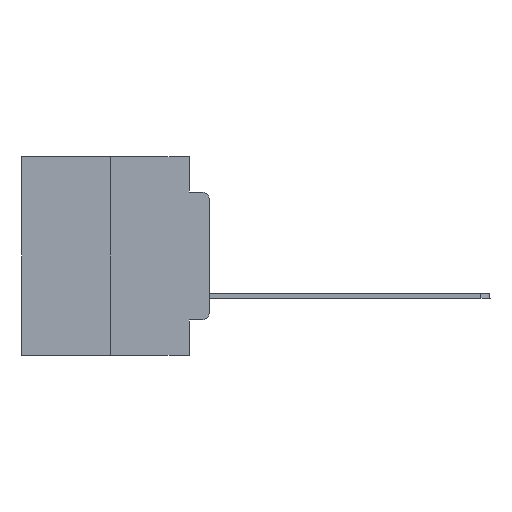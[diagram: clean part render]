
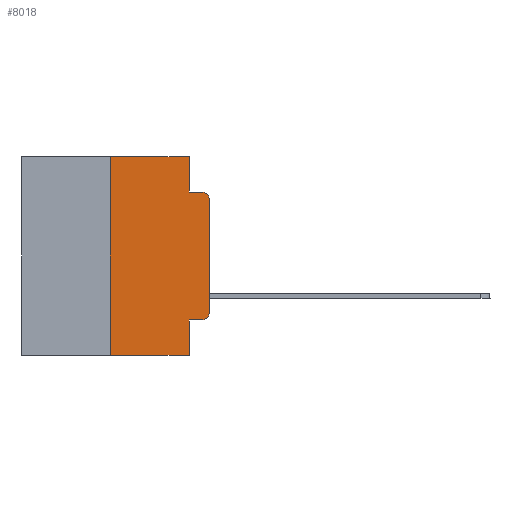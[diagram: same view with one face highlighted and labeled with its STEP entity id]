
A CAD part, left-side view. The second image highlights one B-rep face of the part: STEP entity #8018.
In plain terms, the highlighted planar face has unit normal (-1, 0, 0).
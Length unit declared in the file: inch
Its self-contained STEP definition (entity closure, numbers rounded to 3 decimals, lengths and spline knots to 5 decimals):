
#110 = LINE ( 'NONE', #20699, #1363 ) ;
#920 = EDGE_LOOP ( 'NONE', ( #15787, #13832, #15679, #2842, #12785, #22936, #7145, #8000, #10165, #6004 ) ) ;
#1363 = VECTOR ( 'NONE', #5679, 39.37008 ) ;
#1637 = DIRECTION ( 'NONE',  ( 0., 0., 1. ) ) ;
#1907 = EDGE_CURVE ( 'NONE', #15373, #3671, #4160, .T. ) ;
#2144 = CARTESIAN_POINT ( 'NONE',  ( 0., 0.02, -0.0885 ) ) ;
#2605 = CARTESIAN_POINT ( 'NONE',  ( 0., 0.02, -0.4115 ) ) ;
#2620 = CARTESIAN_POINT ( 'NONE',  ( 0., 0.051, -0.0885 ) ) ;
#2698 = VECTOR ( 'NONE', #14710, 39.37008 ) ;
#2842 = ORIENTED_EDGE ( 'NONE', *, *, #9728, .F. ) ;
#3425 = VERTEX_POINT ( 'NONE', #2605 ) ;
#3671 = VERTEX_POINT ( 'NONE', #13565 ) ;
#4160 = LINE ( 'NONE', #23422, #6907 ) ;
#4455 = VERTEX_POINT ( 'NONE', #24494 ) ;
#4580 = DIRECTION ( 'NONE',  ( 0., -1., 0. ) ) ;
#4675 = VECTOR ( 'NONE', #8907, 39.37008 ) ;
#4723 = DIRECTION ( 'NONE',  ( 0., -1., 0. ) ) ;
#4788 = VERTEX_POINT ( 'NONE', #14912 ) ;
#4839 = AXIS2_PLACEMENT_3D ( 'NONE', #7687, #7604, #5949 ) ;
#5307 = LINE ( 'NONE', #22764, #11201 ) ;
#5679 = DIRECTION ( 'NONE',  ( 0., 0., -1. ) ) ;
#5792 = CARTESIAN_POINT ( 'NONE',  ( 0., 0.25, -0.5 ) ) ;
#5949 = DIRECTION ( 'NONE',  ( 0., 0., -1. ) ) ;
#6004 = ORIENTED_EDGE ( 'NONE', *, *, #6723, .T. ) ;
#6352 = CARTESIAN_POINT ( 'NONE',  ( 0., 0.051, -0.4115 ) ) ;
#6611 = CARTESIAN_POINT ( 'NONE',  ( 0., 0.473, 0. ) ) ;
#6723 = EDGE_CURVE ( 'NONE', #3425, #19789, #13620, .T. ) ;
#6907 = VECTOR ( 'NONE', #13314, 39.37008 ) ;
#7145 = ORIENTED_EDGE ( 'NONE', *, *, #1907, .T. ) ;
#7290 = LINE ( 'NONE', #14428, #11926 ) ;
#7604 = DIRECTION ( 'NONE',  ( -1., 0., 0. ) ) ;
#7687 = CARTESIAN_POINT ( 'NONE',  ( 0., 0.02, -0.3915 ) ) ;
#8000 = ORIENTED_EDGE ( 'NONE', *, *, #24220, .F. ) ;
#8018 = ADVANCED_FACE ( 'NONE', ( #23528 ), #16498, .F. ) ;
#8704 = DIRECTION ( 'NONE',  ( 0., 0., -1. ) ) ;
#8907 = DIRECTION ( 'NONE',  ( 0., 0., 1. ) ) ;
#9728 = EDGE_CURVE ( 'NONE', #21438, #4788, #5307, .T. ) ;
#10165 = ORIENTED_EDGE ( 'NONE', *, *, #18869, .T. ) ;
#10586 = CARTESIAN_POINT ( 'NONE',  ( 0., 0.051, 0. ) ) ;
#10835 = DIRECTION ( 'NONE',  ( 0., 0., -1. ) ) ;
#10953 = CARTESIAN_POINT ( 'NONE',  ( 0., 0.25, 0. ) ) ;
#10961 = CARTESIAN_POINT ( 'NONE',  ( 0., 0., -0.3915 ) ) ;
#11027 = CARTESIAN_POINT ( 'NONE',  ( 0., 0., -0.1085 ) ) ;
#11164 = CARTESIAN_POINT ( 'NONE',  ( 0., 0.02, -0.1085 ) ) ;
#11201 = VECTOR ( 'NONE', #10835, 39.37008 ) ;
#11926 = VECTOR ( 'NONE', #4723, 39.37008 ) ;
#12785 = ORIENTED_EDGE ( 'NONE', *, *, #19736, .F. ) ;
#13314 = DIRECTION ( 'NONE',  ( 0., -1., 0. ) ) ;
#13565 = CARTESIAN_POINT ( 'NONE',  ( 0., 0.051, -0.5 ) ) ;
#13620 = CIRCLE ( 'NONE', #4839, 0.02 ) ;
#13832 = ORIENTED_EDGE ( 'NONE', *, *, #16430, .T. ) ;
#14428 = CARTESIAN_POINT ( 'NONE',  ( 0., 0.473, 0. ) ) ;
#14657 = CARTESIAN_POINT ( 'NONE',  ( 0., 0.25, 0. ) ) ;
#14710 = DIRECTION ( 'NONE',  ( 0., -1., 0. ) ) ;
#14853 = EDGE_CURVE ( 'NONE', #4788, #22424, #18053, .T. ) ;
#14912 = CARTESIAN_POINT ( 'NONE',  ( 0., 0.051, -0.0885 ) ) ;
#15373 = VERTEX_POINT ( 'NONE', #5792 ) ;
#15411 = DIRECTION ( 'NONE',  ( 0., 0., -1. ) ) ;
#15679 = ORIENTED_EDGE ( 'NONE', *, *, #14853, .F. ) ;
#15787 = ORIENTED_EDGE ( 'NONE', *, *, #25307, .T. ) ;
#16184 = VECTOR ( 'NONE', #1637, 39.37008 ) ;
#16346 = EDGE_CURVE ( 'NONE', #15373, #22776, #23337, .T. ) ;
#16430 = EDGE_CURVE ( 'NONE', #20087, #22424, #16431, .T. ) ;
#16431 = CIRCLE ( 'NONE', #22677, 0.02 ) ;
#16498 = PLANE ( 'NONE',  #22017 ) ;
#16595 = LINE ( 'NONE', #6352, #2698 ) ;
#18053 = LINE ( 'NONE', #2620, #18691 ) ;
#18691 = VECTOR ( 'NONE', #4580, 39.37008 ) ;
#18869 = EDGE_CURVE ( 'NONE', #4455, #3425, #16595, .T. ) ;
#19424 = DIRECTION ( 'NONE',  ( -1., 0., 0. ) ) ;
#19736 = EDGE_CURVE ( 'NONE', #22776, #21438, #7290, .T. ) ;
#19789 = VERTEX_POINT ( 'NONE', #10961 ) ;
#20087 = VERTEX_POINT ( 'NONE', #11027 ) ;
#20345 = DIRECTION ( 'NONE',  ( 1., 0., 0. ) ) ;
#20699 = CARTESIAN_POINT ( 'NONE',  ( 0., 0.051, 0. ) ) ;
#21438 = VERTEX_POINT ( 'NONE', #10586 ) ;
#22017 = AXIS2_PLACEMENT_3D ( 'NONE', #6611, #20345, #8704 ) ;
#22424 = VERTEX_POINT ( 'NONE', #2144 ) ;
#22677 = AXIS2_PLACEMENT_3D ( 'NONE', #11164, #19424, #15411 ) ;
#22764 = CARTESIAN_POINT ( 'NONE',  ( 0., 0.051, 0. ) ) ;
#22776 = VERTEX_POINT ( 'NONE', #10953 ) ;
#22936 = ORIENTED_EDGE ( 'NONE', *, *, #16346, .F. ) ;
#23337 = LINE ( 'NONE', #14657, #4675 ) ;
#23422 = CARTESIAN_POINT ( 'NONE',  ( 0., 0.473, -0.5 ) ) ;
#23528 = FACE_OUTER_BOUND ( 'NONE', #920, .T. ) ;
#24220 = EDGE_CURVE ( 'NONE', #4455, #3671, #110, .T. ) ;
#24494 = CARTESIAN_POINT ( 'NONE',  ( 0., 0.051, -0.4115 ) ) ;
#25307 = EDGE_CURVE ( 'NONE', #19789, #20087, #25548, .T. ) ;
#25548 = LINE ( 'NONE', #25637, #16184 ) ;
#25637 = CARTESIAN_POINT ( 'NONE',  ( 0., 0., 0. ) ) ;
